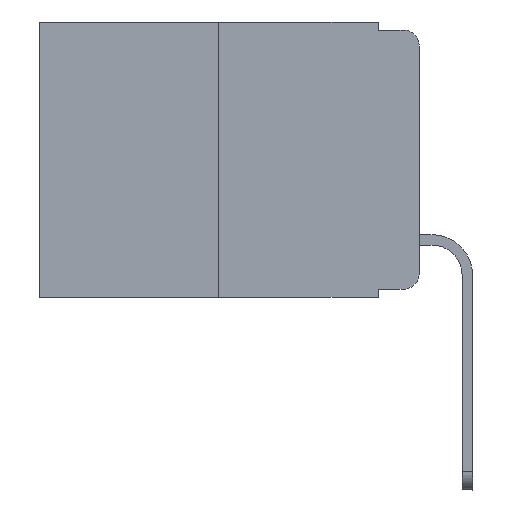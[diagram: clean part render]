
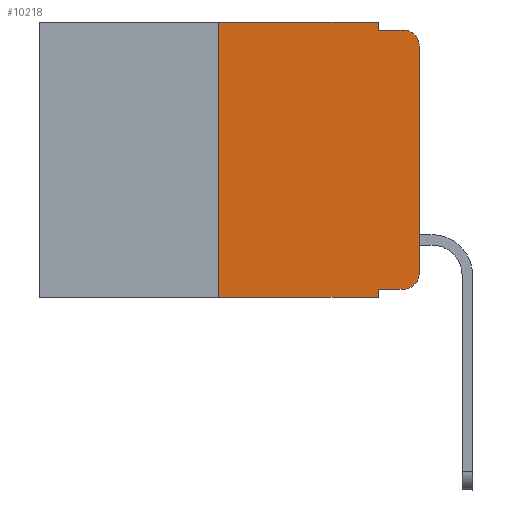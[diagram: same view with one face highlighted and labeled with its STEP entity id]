
A CAD part, left-side view. The second image highlights one B-rep face of the part: STEP entity #10218.
In plain terms, the highlighted planar face has unit normal (-1, 0, 0).
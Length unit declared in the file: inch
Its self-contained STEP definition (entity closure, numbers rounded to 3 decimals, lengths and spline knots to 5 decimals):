
#67 = EDGE_CURVE ( 'NONE', #16165, #7981, #1174, .T. ) ;
#230 = CARTESIAN_POINT ( 'NONE',  ( 0., 0.473, -0.343 ) ) ;
#356 = CARTESIAN_POINT ( 'NONE',  ( 0., 0.051, -0.333 ) ) ;
#518 = EDGE_CURVE ( 'NONE', #8501, #7981, #12368, .T. ) ;
#783 = EDGE_CURVE ( 'NONE', #4516, #11554, #10982, .T. ) ;
#1174 = CIRCLE ( 'NONE', #10394, 0.02 ) ;
#1180 = ORIENTED_EDGE ( 'NONE', *, *, #2502, .F. ) ;
#1240 = VECTOR ( 'NONE', #7275, 39.37008 ) ;
#1735 = LINE ( 'NONE', #15715, #12059 ) ;
#1780 = DIRECTION ( 'NONE',  ( 1., 0., 0. ) ) ;
#1849 = VECTOR ( 'NONE', #11293, 39.37008 ) ;
#1897 = ORIENTED_EDGE ( 'NONE', *, *, #6998, .T. ) ;
#2160 = VECTOR ( 'NONE', #3832, 39.37008 ) ;
#2424 = CARTESIAN_POINT ( 'NONE',  ( 0., 0.051, -0.01 ) ) ;
#2502 = EDGE_CURVE ( 'NONE', #6968, #13834, #2584, .T. ) ;
#2566 = EDGE_CURVE ( 'NONE', #4345, #8557, #9035, .T. ) ;
#2577 = LINE ( 'NONE', #230, #2160 ) ;
#2584 = LINE ( 'NONE', #11647, #10586 ) ;
#2799 = DIRECTION ( 'NONE',  ( 0., 0., -1. ) ) ;
#3055 = DIRECTION ( 'NONE',  ( 0., -1., 0. ) ) ;
#3057 = CARTESIAN_POINT ( 'NONE',  ( 0., 0.02, -0.333 ) ) ;
#3091 = EDGE_CURVE ( 'NONE', #11554, #6647, #1735, .T. ) ;
#3128 = CARTESIAN_POINT ( 'NONE',  ( 0., 0.051, 0. ) ) ;
#3615 = VECTOR ( 'NONE', #5078, 39.37008 ) ;
#3832 = DIRECTION ( 'NONE',  ( 0., -1., 0. ) ) ;
#4084 = DIRECTION ( 'NONE',  ( 0., 0., -1. ) ) ;
#4345 = VERTEX_POINT ( 'NONE', #3057 ) ;
#4516 = VERTEX_POINT ( 'NONE', #12188 ) ;
#4712 = VECTOR ( 'NONE', #9240, 39.37008 ) ;
#5078 = DIRECTION ( 'NONE',  ( 0., -1., 0. ) ) ;
#5276 = PLANE ( 'NONE',  #7961 ) ;
#5383 = CARTESIAN_POINT ( 'NONE',  ( 0., 0.051, -0.343 ) ) ;
#5548 = CARTESIAN_POINT ( 'NONE',  ( 0., 0.051, 0. ) ) ;
#5595 = ORIENTED_EDGE ( 'NONE', *, *, #783, .F. ) ;
#5767 = CARTESIAN_POINT ( 'NONE',  ( 0., 0., -0.313 ) ) ;
#6597 = CARTESIAN_POINT ( 'NONE',  ( 0., 0.25, 0. ) ) ;
#6647 = VERTEX_POINT ( 'NONE', #3128 ) ;
#6968 = VERTEX_POINT ( 'NONE', #10370 ) ;
#6998 = EDGE_CURVE ( 'NONE', #6968, #4345, #14307, .T. ) ;
#7275 = DIRECTION ( 'NONE',  ( 0., 0., 1. ) ) ;
#7296 = ORIENTED_EDGE ( 'NONE', *, *, #3091, .F. ) ;
#7961 = AXIS2_PLACEMENT_3D ( 'NONE', #11506, #1780, #15373 ) ;
#7981 = VERTEX_POINT ( 'NONE', #8865 ) ;
#8501 = VERTEX_POINT ( 'NONE', #10871 ) ;
#8557 = VERTEX_POINT ( 'NONE', #5767 ) ;
#8623 = ORIENTED_EDGE ( 'NONE', *, *, #10452, .T. ) ;
#8865 = CARTESIAN_POINT ( 'NONE',  ( 0., 0.02, -0.01 ) ) ;
#9035 = CIRCLE ( 'NONE', #15838, 0.02 ) ;
#9070 = ORIENTED_EDGE ( 'NONE', *, *, #9582, .T. ) ;
#9240 = DIRECTION ( 'NONE',  ( 0., -1., 0. ) ) ;
#9582 = EDGE_CURVE ( 'NONE', #8557, #16165, #14910, .T. ) ;
#9858 = ORIENTED_EDGE ( 'NONE', *, *, #2566, .T. ) ;
#10031 = DIRECTION ( 'NONE',  ( -1., 0., 0. ) ) ;
#10102 = CARTESIAN_POINT ( 'NONE',  ( 0., 0.02, -0.03 ) ) ;
#10218 = ADVANCED_FACE ( 'NONE', ( #14221 ), #5276, .F. ) ;
#10249 = DIRECTION ( 'NONE',  ( 0., 0., -1. ) ) ;
#10306 = LINE ( 'NONE', #5548, #15238 ) ;
#10370 = CARTESIAN_POINT ( 'NONE',  ( 0., 0.051, -0.333 ) ) ;
#10394 = AXIS2_PLACEMENT_3D ( 'NONE', #10102, #10031, #15105 ) ;
#10452 = EDGE_CURVE ( 'NONE', #4516, #13834, #2577, .T. ) ;
#10491 = ORIENTED_EDGE ( 'NONE', *, *, #67, .T. ) ;
#10586 = VECTOR ( 'NONE', #10249, 39.37008 ) ;
#10871 = CARTESIAN_POINT ( 'NONE',  ( 0., 0.051, -0.01 ) ) ;
#10982 = LINE ( 'NONE', #13498, #1240 ) ;
#11221 = CARTESIAN_POINT ( 'NONE',  ( 0., 0., 0. ) ) ;
#11293 = DIRECTION ( 'NONE',  ( 0., 0., 1. ) ) ;
#11506 = CARTESIAN_POINT ( 'NONE',  ( 0., 0.473, 0. ) ) ;
#11554 = VERTEX_POINT ( 'NONE', #6597 ) ;
#11647 = CARTESIAN_POINT ( 'NONE',  ( 0., 0.051, 0. ) ) ;
#12059 = VECTOR ( 'NONE', #3055, 39.37008 ) ;
#12188 = CARTESIAN_POINT ( 'NONE',  ( 0., 0.25, -0.343 ) ) ;
#12368 = LINE ( 'NONE', #2424, #3615 ) ;
#13498 = CARTESIAN_POINT ( 'NONE',  ( 0., 0.25, 0. ) ) ;
#13558 = ORIENTED_EDGE ( 'NONE', *, *, #518, .F. ) ;
#13834 = VERTEX_POINT ( 'NONE', #5383 ) ;
#14020 = CARTESIAN_POINT ( 'NONE',  ( 0., 0.02, -0.313 ) ) ;
#14221 = FACE_OUTER_BOUND ( 'NONE', #14872, .T. ) ;
#14307 = LINE ( 'NONE', #356, #4712 ) ;
#14400 = CARTESIAN_POINT ( 'NONE',  ( 0., 0., -0.03 ) ) ;
#14720 = ORIENTED_EDGE ( 'NONE', *, *, #14921, .F. ) ;
#14872 = EDGE_LOOP ( 'NONE', ( #9070, #10491, #13558, #14720, #7296, #5595, #8623, #1180, #1897, #9858 ) ) ;
#14910 = LINE ( 'NONE', #11221, #1849 ) ;
#14921 = EDGE_CURVE ( 'NONE', #6647, #8501, #10306, .T. ) ;
#15105 = DIRECTION ( 'NONE',  ( 0., 0., -1. ) ) ;
#15238 = VECTOR ( 'NONE', #2799, 39.37008 ) ;
#15342 = DIRECTION ( 'NONE',  ( -1., 0., 0. ) ) ;
#15373 = DIRECTION ( 'NONE',  ( 0., 0., -1. ) ) ;
#15715 = CARTESIAN_POINT ( 'NONE',  ( 0., 0.473, 0. ) ) ;
#15838 = AXIS2_PLACEMENT_3D ( 'NONE', #14020, #15342, #4084 ) ;
#16165 = VERTEX_POINT ( 'NONE', #14400 ) ;
